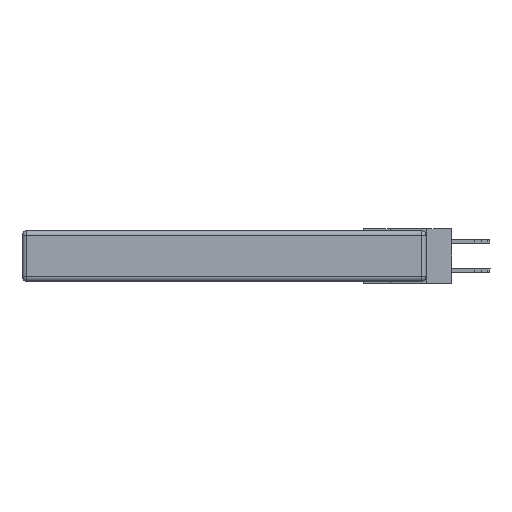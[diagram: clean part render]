
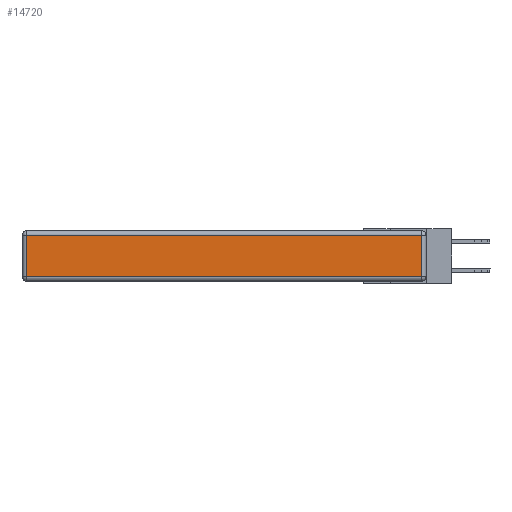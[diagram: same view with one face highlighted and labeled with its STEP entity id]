
A CAD part, left-side view. The second image highlights one B-rep face of the part: STEP entity #14720.
In plain terms, the highlighted planar face has unit normal (-1, 0, 0).
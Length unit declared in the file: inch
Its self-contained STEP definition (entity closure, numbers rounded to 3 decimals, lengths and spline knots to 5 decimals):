
#317 = PLANE ( 'NONE',  #19892 ) ;
#3658 = FACE_OUTER_BOUND ( 'NONE', #8994, .T. ) ;
#5162 = LINE ( 'NONE', #18781, #25245 ) ;
#6960 = ORIENTED_EDGE ( 'NONE', *, *, #27110, .T. ) ;
#7502 = DIRECTION ( 'NONE',  ( 0., 0., 1. ) ) ;
#7541 = DIRECTION ( 'NONE',  ( 0., -1., 0. ) ) ;
#8513 = DIRECTION ( 'NONE',  ( 0., 0., -1. ) ) ;
#8994 = EDGE_LOOP ( 'NONE', ( #9034, #22380, #6960, #22763 ) ) ;
#9034 = ORIENTED_EDGE ( 'NONE', *, *, #26500, .T. ) ;
#9291 = CARTESIAN_POINT ( 'NONE',  ( 0., 2.72, -0.03 ) ) ;
#9632 = CARTESIAN_POINT ( 'NONE',  ( 0., 0.03, -0.343 ) ) ;
#11196 = LINE ( 'NONE', #25928, #16255 ) ;
#12319 = DIRECTION ( 'NONE',  ( 0., 1., 0. ) ) ;
#12927 = LINE ( 'NONE', #20610, #22620 ) ;
#13337 = DIRECTION ( 'NONE',  ( 0., 0., 1. ) ) ;
#13817 = LINE ( 'NONE', #9632, #25509 ) ;
#14720 = ADVANCED_FACE ( 'NONE', ( #3658 ), #317, .T. ) ;
#16255 = VECTOR ( 'NONE', #8513, 39.37008 ) ;
#17510 = VERTEX_POINT ( 'NONE', #27453 ) ;
#18781 = CARTESIAN_POINT ( 'NONE',  ( 0., 2.75, -0.03 ) ) ;
#19036 = VERTEX_POINT ( 'NONE', #27388 ) ;
#19703 = CARTESIAN_POINT ( 'NONE',  ( 0., 0.03, -0.313 ) ) ;
#19892 = AXIS2_PLACEMENT_3D ( 'NONE', #24026, #25908, #13337 ) ;
#20610 = CARTESIAN_POINT ( 'NONE',  ( 0., 0., -0.313 ) ) ;
#21256 = VERTEX_POINT ( 'NONE', #19703 ) ;
#21939 = EDGE_CURVE ( 'NONE', #26825, #17510, #11196, .T. ) ;
#22380 = ORIENTED_EDGE ( 'NONE', *, *, #24498, .T. ) ;
#22620 = VECTOR ( 'NONE', #7541, 39.37008 ) ;
#22763 = ORIENTED_EDGE ( 'NONE', *, *, #21939, .T. ) ;
#24026 = CARTESIAN_POINT ( 'NONE',  ( 0., 0., -0.343 ) ) ;
#24498 = EDGE_CURVE ( 'NONE', #21256, #19036, #13817, .T. ) ;
#25245 = VECTOR ( 'NONE', #12319, 39.37008 ) ;
#25509 = VECTOR ( 'NONE', #7502, 39.37008 ) ;
#25908 = DIRECTION ( 'NONE',  ( -1., 0., 0. ) ) ;
#25928 = CARTESIAN_POINT ( 'NONE',  ( 0., 2.72, -0.343 ) ) ;
#26500 = EDGE_CURVE ( 'NONE', #17510, #21256, #12927, .T. ) ;
#26825 = VERTEX_POINT ( 'NONE', #9291 ) ;
#27110 = EDGE_CURVE ( 'NONE', #19036, #26825, #5162, .T. ) ;
#27388 = CARTESIAN_POINT ( 'NONE',  ( 0., 0.03, -0.03 ) ) ;
#27453 = CARTESIAN_POINT ( 'NONE',  ( 0., 2.72, -0.313 ) ) ;
